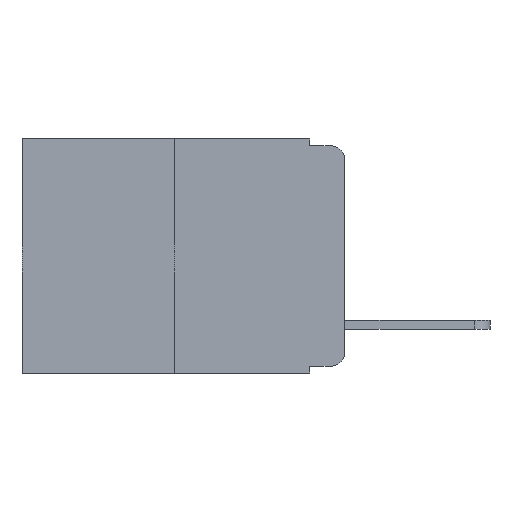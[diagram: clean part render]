
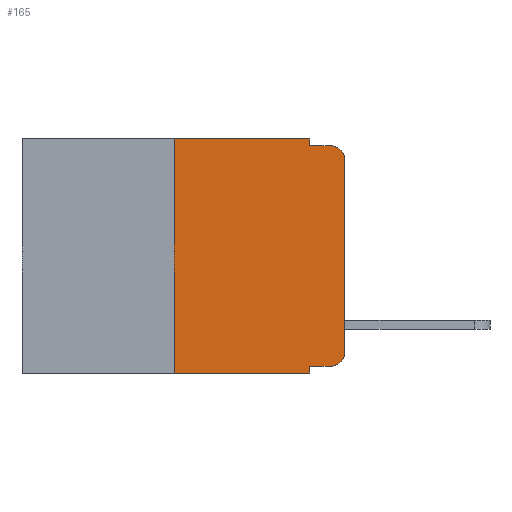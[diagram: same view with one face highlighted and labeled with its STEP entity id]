
A CAD part, left-side view. The second image highlights one B-rep face of the part: STEP entity #165.
In plain terms, the highlighted planar face has unit normal (-1, 0, 0).
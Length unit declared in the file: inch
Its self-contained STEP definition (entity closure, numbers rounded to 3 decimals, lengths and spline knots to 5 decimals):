
#165 = ADVANCED_FACE ( 'NONE', ( #2963 ), #3882, .F. ) ;
#175 = VECTOR ( 'NONE', #9739, 39.37008 ) ;
#240 = DIRECTION ( 'NONE',  ( 1., 0., 0. ) ) ;
#253 = VERTEX_POINT ( 'NONE', #15624 ) ;
#343 = DIRECTION ( 'NONE',  ( 0., 0., -1. ) ) ;
#411 = VERTEX_POINT ( 'NONE', #13330 ) ;
#581 = CARTESIAN_POINT ( 'NONE',  ( 0., 0.051, -0.333 ) ) ;
#748 = DIRECTION ( 'NONE',  ( 0., 0., -1. ) ) ;
#810 = DIRECTION ( 'NONE',  ( 0., -1., 0. ) ) ;
#834 = VERTEX_POINT ( 'NONE', #8859 ) ;
#934 = CARTESIAN_POINT ( 'NONE',  ( 0., 0.051, 0. ) ) ;
#1502 = EDGE_CURVE ( 'NONE', #411, #13098, #17311, .T. ) ;
#1722 = DIRECTION ( 'NONE',  ( -1., 0., 0. ) ) ;
#1889 = AXIS2_PLACEMENT_3D ( 'NONE', #18657, #18660, #18672 ) ;
#2116 = LINE ( 'NONE', #934, #15279 ) ;
#2963 = FACE_OUTER_BOUND ( 'NONE', #3624, .T. ) ;
#3020 = EDGE_CURVE ( 'NONE', #4658, #253, #4314, .T. ) ;
#3032 = VECTOR ( 'NONE', #5572, 39.37008 ) ;
#3198 = VECTOR ( 'NONE', #16389, 39.37008 ) ;
#3352 = ORIENTED_EDGE ( 'NONE', *, *, #11386, .F. ) ;
#3359 = VECTOR ( 'NONE', #810, 39.37008 ) ;
#3554 = CARTESIAN_POINT ( 'NONE',  ( 0., 0.473, 0. ) ) ;
#3624 = EDGE_LOOP ( 'NONE', ( #17435, #17826, #5833, #16222, #14083, #3352, #17069, #10191, #4306, #4595 ) ) ;
#3708 = CARTESIAN_POINT ( 'NONE',  ( 0., 0.25, -0.343 ) ) ;
#3732 = LINE ( 'NONE', #15938, #3198 ) ;
#3882 = PLANE ( 'NONE',  #9663 ) ;
#4306 = ORIENTED_EDGE ( 'NONE', *, *, #7402, .T. ) ;
#4314 = CIRCLE ( 'NONE', #7423, 0.02 ) ;
#4518 = LINE ( 'NONE', #11776, #15334 ) ;
#4595 = ORIENTED_EDGE ( 'NONE', *, *, #3020, .T. ) ;
#4658 = VERTEX_POINT ( 'NONE', #18863 ) ;
#4828 = EDGE_CURVE ( 'NONE', #253, #411, #3732, .T. ) ;
#4927 = VERTEX_POINT ( 'NONE', #9079 ) ;
#5572 = DIRECTION ( 'NONE',  ( 0., -1., 0. ) ) ;
#5833 = ORIENTED_EDGE ( 'NONE', *, *, #15948, .F. ) ;
#6657 = VECTOR ( 'NONE', #16895, 39.37008 ) ;
#7377 = LINE ( 'NONE', #11606, #3032 ) ;
#7402 = EDGE_CURVE ( 'NONE', #8656, #4658, #12657, .T. ) ;
#7423 = AXIS2_PLACEMENT_3D ( 'NONE', #12093, #1722, #10674 ) ;
#7501 = CARTESIAN_POINT ( 'NONE',  ( 0., 0.051, -0.333 ) ) ;
#8656 = VERTEX_POINT ( 'NONE', #581 ) ;
#8859 = CARTESIAN_POINT ( 'NONE',  ( 0., 0.051, -0.343 ) ) ;
#9079 = CARTESIAN_POINT ( 'NONE',  ( 0., 0.051, 0. ) ) ;
#9360 = VERTEX_POINT ( 'NONE', #3708 ) ;
#9663 = AXIS2_PLACEMENT_3D ( 'NONE', #3554, #240, #343 ) ;
#9739 = DIRECTION ( 'NONE',  ( 0., -1., 0. ) ) ;
#9957 = VERTEX_POINT ( 'NONE', #12376 ) ;
#10008 = CARTESIAN_POINT ( 'NONE',  ( 0., 0.25, 0. ) ) ;
#10191 = ORIENTED_EDGE ( 'NONE', *, *, #10417, .F. ) ;
#10417 = EDGE_CURVE ( 'NONE', #8656, #834, #4518, .T. ) ;
#10674 = DIRECTION ( 'NONE',  ( 0., 0., -1. ) ) ;
#11386 = EDGE_CURVE ( 'NONE', #9360, #9957, #18770, .T. ) ;
#11606 = CARTESIAN_POINT ( 'NONE',  ( 0., 0.473, 0. ) ) ;
#11776 = CARTESIAN_POINT ( 'NONE',  ( 0., 0.051, 0. ) ) ;
#11831 = CARTESIAN_POINT ( 'NONE',  ( 0., 0.473, -0.343 ) ) ;
#12046 = LINE ( 'NONE', #11831, #3359 ) ;
#12093 = CARTESIAN_POINT ( 'NONE',  ( 0., 0.02, -0.313 ) ) ;
#12107 = VERTEX_POINT ( 'NONE', #15379 ) ;
#12376 = CARTESIAN_POINT ( 'NONE',  ( 0., 0.25, 0. ) ) ;
#12657 = LINE ( 'NONE', #7501, #175 ) ;
#13098 = VERTEX_POINT ( 'NONE', #18763 ) ;
#13330 = CARTESIAN_POINT ( 'NONE',  ( 0., 0., -0.03 ) ) ;
#14083 = ORIENTED_EDGE ( 'NONE', *, *, #16661, .F. ) ;
#14139 = EDGE_CURVE ( 'NONE', #4927, #12107, #2116, .T. ) ;
#15279 = VECTOR ( 'NONE', #17293, 39.37008 ) ;
#15301 = VECTOR ( 'NONE', #15575, 39.37008 ) ;
#15334 = VECTOR ( 'NONE', #748, 39.37008 ) ;
#15379 = CARTESIAN_POINT ( 'NONE',  ( 0., 0.051, -0.01 ) ) ;
#15412 = EDGE_CURVE ( 'NONE', #9360, #834, #12046, .T. ) ;
#15547 = CARTESIAN_POINT ( 'NONE',  ( 0., 0.051, -0.01 ) ) ;
#15575 = DIRECTION ( 'NONE',  ( 0., 0., 1. ) ) ;
#15624 = CARTESIAN_POINT ( 'NONE',  ( 0., 0., -0.313 ) ) ;
#15938 = CARTESIAN_POINT ( 'NONE',  ( 0., 0., 0. ) ) ;
#15948 = EDGE_CURVE ( 'NONE', #12107, #13098, #17889, .T. ) ;
#16222 = ORIENTED_EDGE ( 'NONE', *, *, #14139, .F. ) ;
#16389 = DIRECTION ( 'NONE',  ( 0., 0., 1. ) ) ;
#16661 = EDGE_CURVE ( 'NONE', #9957, #4927, #7377, .T. ) ;
#16895 = DIRECTION ( 'NONE',  ( 0., -1., 0. ) ) ;
#17069 = ORIENTED_EDGE ( 'NONE', *, *, #15412, .T. ) ;
#17293 = DIRECTION ( 'NONE',  ( 0., 0., -1. ) ) ;
#17311 = CIRCLE ( 'NONE', #1889, 0.02 ) ;
#17435 = ORIENTED_EDGE ( 'NONE', *, *, #4828, .T. ) ;
#17826 = ORIENTED_EDGE ( 'NONE', *, *, #1502, .T. ) ;
#17889 = LINE ( 'NONE', #15547, #6657 ) ;
#18657 = CARTESIAN_POINT ( 'NONE',  ( 0., 0.02, -0.03 ) ) ;
#18660 = DIRECTION ( 'NONE',  ( -1., 0., 0. ) ) ;
#18672 = DIRECTION ( 'NONE',  ( 0., 0., -1. ) ) ;
#18763 = CARTESIAN_POINT ( 'NONE',  ( 0., 0.02, -0.01 ) ) ;
#18770 = LINE ( 'NONE', #10008, #15301 ) ;
#18863 = CARTESIAN_POINT ( 'NONE',  ( 0., 0.02, -0.333 ) ) ;
